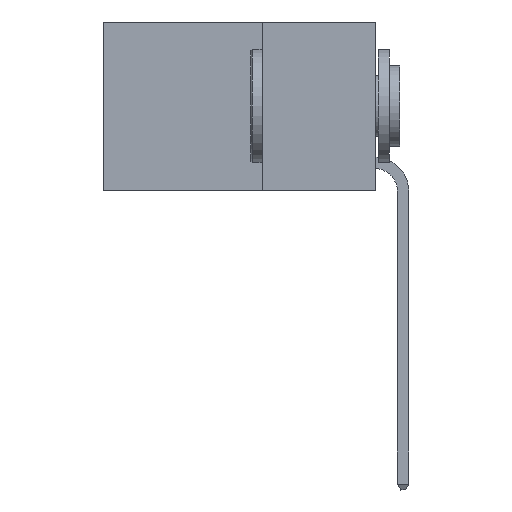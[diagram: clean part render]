
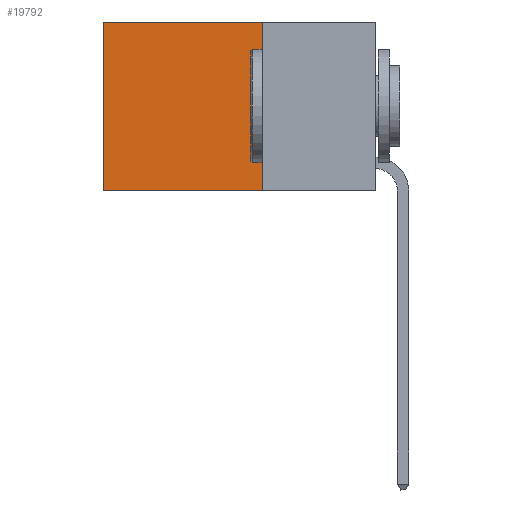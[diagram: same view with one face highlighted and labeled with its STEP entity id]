
A CAD part, left-side view. The second image highlights one B-rep face of the part: STEP entity #19792.
In plain terms, the highlighted planar face has unit normal (-1, 0, 0).
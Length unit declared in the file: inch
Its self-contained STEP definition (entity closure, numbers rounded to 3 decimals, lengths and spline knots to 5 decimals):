
#496 = DIRECTION ( 'NONE',  ( 0., 1., 0. ) ) ;
#1602 = LINE ( 'NONE', #27633, #12187 ) ;
#2000 = PLANE ( 'NONE',  #15180 ) ;
#2209 = VERTEX_POINT ( 'NONE', #19986 ) ;
#3832 = LINE ( 'NONE', #24908, #30267 ) ;
#4561 = EDGE_LOOP ( 'NONE', ( #17063, #10174, #14281, #17038 ) ) ;
#6277 = EDGE_CURVE ( 'NONE', #6936, #8087, #1602, .T. ) ;
#6936 = VERTEX_POINT ( 'NONE', #19633 ) ;
#8087 = VERTEX_POINT ( 'NONE', #23449 ) ;
#8963 = CARTESIAN_POINT ( 'NONE',  ( 0.2625, 0.25, 0. ) ) ;
#9163 = CARTESIAN_POINT ( 'NONE',  ( 0.2625, 0.25, 0. ) ) ;
#10174 = ORIENTED_EDGE ( 'NONE', *, *, #6277, .F. ) ;
#10964 = EDGE_CURVE ( 'NONE', #2209, #8087, #3832, .T. ) ;
#12187 = VECTOR ( 'NONE', #28097, 39.37008 ) ;
#13429 = LINE ( 'NONE', #8963, #19140 ) ;
#13804 = CARTESIAN_POINT ( 'NONE',  ( 0.2625, 0.25, 0. ) ) ;
#14281 = ORIENTED_EDGE ( 'NONE', *, *, #21510, .F. ) ;
#15180 = AXIS2_PLACEMENT_3D ( 'NONE', #9163, #27723, #16120 ) ;
#16120 = DIRECTION ( 'NONE',  ( 0., 0., -1. ) ) ;
#16239 = VERTEX_POINT ( 'NONE', #13804 ) ;
#16909 = LINE ( 'NONE', #19258, #28842 ) ;
#17038 = ORIENTED_EDGE ( 'NONE', *, *, #26082, .T. ) ;
#17063 = ORIENTED_EDGE ( 'NONE', *, *, #10964, .T. ) ;
#19140 = VECTOR ( 'NONE', #20731, 39.37008 ) ;
#19258 = CARTESIAN_POINT ( 'NONE',  ( 0.2625, 0.25, 0. ) ) ;
#19633 = CARTESIAN_POINT ( 'NONE',  ( 0.2625, 0.25, -0.37 ) ) ;
#19792 = ADVANCED_FACE ( 'NONE', ( #23417 ), #2000, .F. ) ;
#19986 = CARTESIAN_POINT ( 'NONE',  ( 0.2625, 0.6, 0. ) ) ;
#20731 = DIRECTION ( 'NONE',  ( 0., 0., -1. ) ) ;
#21510 = EDGE_CURVE ( 'NONE', #16239, #6936, #13429, .T. ) ;
#22101 = DIRECTION ( 'NONE',  ( 0., 0., -1. ) ) ;
#23417 = FACE_OUTER_BOUND ( 'NONE', #4561, .T. ) ;
#23449 = CARTESIAN_POINT ( 'NONE',  ( 0.2625, 0.6, -0.37 ) ) ;
#24908 = CARTESIAN_POINT ( 'NONE',  ( 0.2625, 0.6, 0. ) ) ;
#26082 = EDGE_CURVE ( 'NONE', #16239, #2209, #16909, .T. ) ;
#27633 = CARTESIAN_POINT ( 'NONE',  ( 0.2625, 0.25, -0.37 ) ) ;
#27723 = DIRECTION ( 'NONE',  ( 1., 0., 0. ) ) ;
#28097 = DIRECTION ( 'NONE',  ( 0., 1., 0. ) ) ;
#28842 = VECTOR ( 'NONE', #496, 39.37008 ) ;
#30267 = VECTOR ( 'NONE', #22101, 39.37008 ) ;
